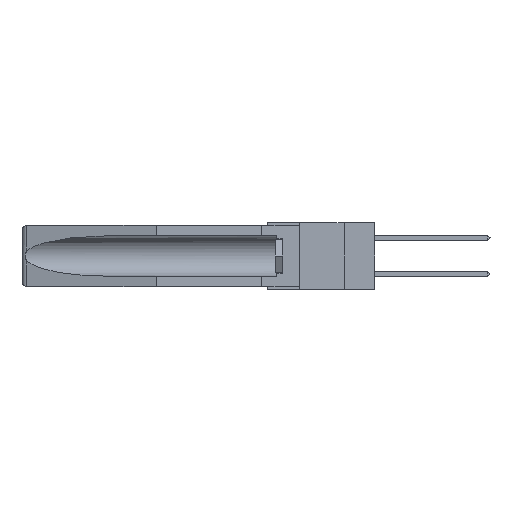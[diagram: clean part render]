
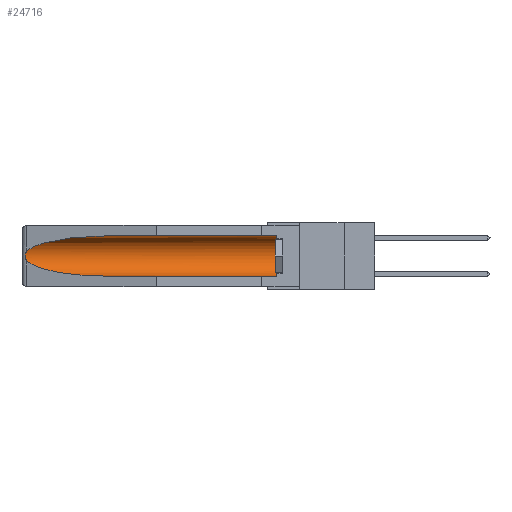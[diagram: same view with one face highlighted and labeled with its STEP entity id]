
A CAD part, left-side view. The second image highlights one B-rep face of the part: STEP entity #24716.
In plain terms, the highlighted cylindrical face has radius 2.857 mm (diameter 5.715 mm), a partial arc.
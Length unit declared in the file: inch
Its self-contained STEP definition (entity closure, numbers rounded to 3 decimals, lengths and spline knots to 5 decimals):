
#7 = CARTESIAN_POINT ( 'NONE',  ( 0.155, -0.30754, -0.284 ) ) ;
#162 = B_SPLINE_CURVE_WITH_KNOTS ( 'NONE', 3,
 ( #28654, #5838, #15810, #8199, #13214, #10987, #16018, #29004, #13330, #31558 ),
 .UNSPECIFIED., .F., .F.,
 ( 4, 2, 2, 2, 4 ),
 ( 0., 0.00029, 0.00058, 0.00087, 0.00117 ),
 .UNSPECIFIED. ) ;
#389 = DIRECTION ( 'NONE',  ( 0., -1., 0. ) ) ;
#847 = CIRCLE ( 'NONE', #21077, 0.1125 ) ;
#1104 = FACE_OUTER_BOUND ( 'NONE', #7961, .T. ) ;
#1195 = VERTEX_POINT ( 'NONE', #27857 ) ;
#1610 = CARTESIAN_POINT ( 'NONE',  ( 0.155, 1.07973, -0.284 ) ) ;
#1719 = CARTESIAN_POINT ( 'NONE',  ( 0.21114, 1.30732, -0.284 ) ) ;
#2587 = DIRECTION ( 'NONE',  ( 0., 1., 0. ) ) ;
#2682 = CARTESIAN_POINT ( 'NONE',  ( 0.26537, 1.52718, -0.14972 ) ) ;
#4110 = VERTEX_POINT ( 'NONE', #22679 ) ;
#5838 = CARTESIAN_POINT ( 'NONE',  ( 0.26597, 1.52961, -0.15275 ) ) ;
#6007 = ORIENTED_EDGE ( 'NONE', *, *, #13263, .T. ) ;
#6926 = DIRECTION ( 'NONE',  ( 0., 1., 0. ) ) ;
#7228 = LINE ( 'NONE', #7, #13173 ) ;
#7747 =( BOUNDED_CURVE ( )  B_SPLINE_CURVE ( 3, ( #9090, #19524, #1719, #1610 ),
 .UNSPECIFIED., .F., .F. ) 
 B_SPLINE_CURVE_WITH_KNOTS ( ( 4, 4 ),
 ( 0.1948, 1.5708 ),
 .UNSPECIFIED. ) 
 CURVE ( )  GEOMETRIC_REPRESENTATION_ITEM ( )  RATIONAL_B_SPLINE_CURVE ( ( 1., 0.848, 0.848, 1. ) ) 
 REPRESENTATION_ITEM ( '' )  );
#7961 = EDGE_LOOP ( 'NONE', ( #6007, #23052, #8666, #29275, #21678, #16694 ) ) ;
#8199 = CARTESIAN_POINT ( 'NONE',  ( 0.2673, 1.5327, -0.16383 ) ) ;
#8278 = CYLINDRICAL_SURFACE ( 'NONE', #11869, 0.1125 ) ;
#8603 = VERTEX_POINT ( 'NONE', #2682 ) ;
#8666 = ORIENTED_EDGE ( 'NONE', *, *, #22341, .T. ) ;
#9090 = CARTESIAN_POINT ( 'NONE',  ( 0.26537, 1.52718, -0.19328 ) ) ;
#9352 = CARTESIAN_POINT ( 'NONE',  ( 0.155, -0.30754, -0.059 ) ) ;
#10987 = CARTESIAN_POINT ( 'NONE',  ( 0.2675, 1.53308, -0.17534 ) ) ;
#11313 = VERTEX_POINT ( 'NONE', #25309 ) ;
#11376 = LINE ( 'NONE', #9352, #19402 ) ;
#11869 = AXIS2_PLACEMENT_3D ( 'NONE', #18407, #26279, #29589 ) ;
#12533 = EDGE_CURVE ( 'NONE', #1195, #29774, #11376, .T. ) ;
#13173 = VECTOR ( 'NONE', #2587, 39.37008 ) ;
#13214 = CARTESIAN_POINT ( 'NONE',  ( 0.2675, 1.53308, -0.16763 ) ) ;
#13263 = EDGE_CURVE ( 'NONE', #29774, #8603, #30029, .T. ) ;
#13330 = CARTESIAN_POINT ( 'NONE',  ( 0.26597, 1.5296, -0.19026 ) ) ;
#14228 = VERTEX_POINT ( 'NONE', #33175 ) ;
#15810 = CARTESIAN_POINT ( 'NONE',  ( 0.26654, 1.53092, -0.15636 ) ) ;
#16018 = CARTESIAN_POINT ( 'NONE',  ( 0.2673, 1.53269, -0.17917 ) ) ;
#16694 = ORIENTED_EDGE ( 'NONE', *, *, #12533, .T. ) ;
#17663 = CARTESIAN_POINT ( 'NONE',  ( 0.25451, 1.48313, -0.09465 ) ) ;
#18407 = CARTESIAN_POINT ( 'NONE',  ( 0.155, -0.30754, -0.1715 ) ) ;
#19402 = VECTOR ( 'NONE', #6926, 39.37008 ) ;
#19418 = CARTESIAN_POINT ( 'NONE',  ( 0.155, 1.07973, -0.059 ) ) ;
#19524 = CARTESIAN_POINT ( 'NONE',  ( 0.25451, 1.48313, -0.24835 ) ) ;
#21077 = AXIS2_PLACEMENT_3D ( 'NONE', #23714, #389, #26287 ) ;
#21678 = ORIENTED_EDGE ( 'NONE', *, *, #22056, .T. ) ;
#22056 = EDGE_CURVE ( 'NONE', #4110, #1195, #847, .T. ) ;
#22341 = EDGE_CURVE ( 'NONE', #11313, #14228, #7747, .T. ) ;
#22679 = CARTESIAN_POINT ( 'NONE',  ( 0.155, 0.126, -0.284 ) ) ;
#22841 = CARTESIAN_POINT ( 'NONE',  ( 0.26537, 1.52718, -0.14972 ) ) ;
#23041 = EDGE_CURVE ( 'NONE', #4110, #14228, #7228, .T. ) ;
#23052 = ORIENTED_EDGE ( 'NONE', *, *, #26756, .T. ) ;
#23714 = CARTESIAN_POINT ( 'NONE',  ( 0.155, 0.126, -0.1715 ) ) ;
#24716 = ADVANCED_FACE ( 'NONE', ( #1104 ), #8278, .F. ) ;
#25309 = CARTESIAN_POINT ( 'NONE',  ( 0.26537, 1.52718, -0.19328 ) ) ;
#26279 = DIRECTION ( 'NONE',  ( 0., 1., 0. ) ) ;
#26287 = DIRECTION ( 'NONE',  ( 0., 0., 1. ) ) ;
#26756 = EDGE_CURVE ( 'NONE', #8603, #11313, #162, .T. ) ;
#27857 = CARTESIAN_POINT ( 'NONE',  ( 0.155, 0.126, -0.059 ) ) ;
#28654 = CARTESIAN_POINT ( 'NONE',  ( 0.26537, 1.52718, -0.14972 ) ) ;
#29004 = CARTESIAN_POINT ( 'NONE',  ( 0.26655, 1.53094, -0.18657 ) ) ;
#29275 = ORIENTED_EDGE ( 'NONE', *, *, #23041, .F. ) ;
#29589 = DIRECTION ( 'NONE',  ( 0., 0., 1. ) ) ;
#29774 = VERTEX_POINT ( 'NONE', #19418 ) ;
#30029 =( BOUNDED_CURVE ( )  B_SPLINE_CURVE ( 3, ( #30625, #30189, #17663, #22841 ),
 .UNSPECIFIED., .F., .F. ) 
 B_SPLINE_CURVE_WITH_KNOTS ( ( 4, 4 ),
 ( 4.71239, 6.08839 ),
 .UNSPECIFIED. ) 
 CURVE ( )  GEOMETRIC_REPRESENTATION_ITEM ( )  RATIONAL_B_SPLINE_CURVE ( ( 1., 0.848, 0.848, 1. ) ) 
 REPRESENTATION_ITEM ( '' )  );
#30189 = CARTESIAN_POINT ( 'NONE',  ( 0.21114, 1.30732, -0.059 ) ) ;
#30625 = CARTESIAN_POINT ( 'NONE',  ( 0.155, 1.07973, -0.059 ) ) ;
#31558 = CARTESIAN_POINT ( 'NONE',  ( 0.26537, 1.52718, -0.19328 ) ) ;
#33175 = CARTESIAN_POINT ( 'NONE',  ( 0.155, 1.07973, -0.284 ) ) ;
